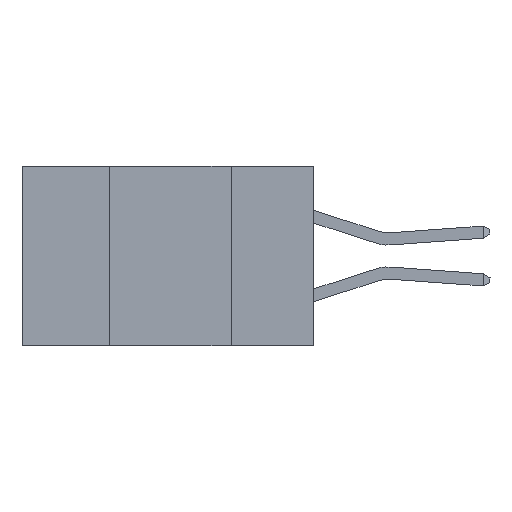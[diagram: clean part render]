
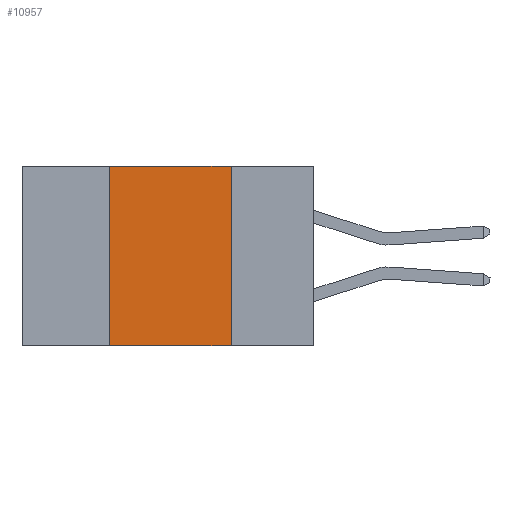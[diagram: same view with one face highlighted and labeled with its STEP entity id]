
A CAD part, left-side view. The second image highlights one B-rep face of the part: STEP entity #10957.
In plain terms, the highlighted planar face has unit normal (-1, 0, 0).
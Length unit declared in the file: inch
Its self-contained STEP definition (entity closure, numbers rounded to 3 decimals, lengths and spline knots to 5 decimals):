
#966 = DIRECTION ( 'NONE',  ( 0., 0., -1. ) ) ;
#1144 = ORIENTED_EDGE ( 'NONE', *, *, #2001, .F. ) ;
#1192 = AXIS2_PLACEMENT_3D ( 'NONE', #4629, #12158, #5756 ) ;
#1366 = CARTESIAN_POINT ( 'NONE',  ( 0., 0.6, 0. ) ) ;
#1712 = DIRECTION ( 'NONE',  ( 0., 0., 1. ) ) ;
#2001 = EDGE_CURVE ( 'NONE', #13180, #4942, #3575, .T. ) ;
#2554 = FACE_OUTER_BOUND ( 'NONE', #12454, .T. ) ;
#3108 = LINE ( 'NONE', #6059, #14188 ) ;
#3410 = VECTOR ( 'NONE', #3708, 39.37008 ) ;
#3421 = VERTEX_POINT ( 'NONE', #8029 ) ;
#3575 = LINE ( 'NONE', #8873, #12205 ) ;
#3578 = CARTESIAN_POINT ( 'NONE',  ( 0., 0.17, -0.37 ) ) ;
#3708 = DIRECTION ( 'NONE',  ( 0., -1., 0. ) ) ;
#3716 = ORIENTED_EDGE ( 'NONE', *, *, #11141, .T. ) ;
#4629 = CARTESIAN_POINT ( 'NONE',  ( 0., 0.6, 0. ) ) ;
#4942 = VERTEX_POINT ( 'NONE', #3578 ) ;
#5756 = DIRECTION ( 'NONE',  ( 0., 0., -1. ) ) ;
#6059 = CARTESIAN_POINT ( 'NONE',  ( 0., 0.6, -0.37 ) ) ;
#6244 = VECTOR ( 'NONE', #1712, 39.37008 ) ;
#6292 = CARTESIAN_POINT ( 'NONE',  ( 0., 0.42, 0. ) ) ;
#6396 = LINE ( 'NONE', #1366, #3410 ) ;
#7393 = CARTESIAN_POINT ( 'NONE',  ( 0., 0.17, 0. ) ) ;
#8029 = CARTESIAN_POINT ( 'NONE',  ( 0., 0.42, 0. ) ) ;
#8271 = DIRECTION ( 'NONE',  ( 0., -1., 0. ) ) ;
#8629 = CARTESIAN_POINT ( 'NONE',  ( 0., 0.42, -0.37 ) ) ;
#8873 = CARTESIAN_POINT ( 'NONE',  ( 0., 0.17, 0. ) ) ;
#9427 = EDGE_CURVE ( 'NONE', #3421, #13180, #6396, .T. ) ;
#9950 = ORIENTED_EDGE ( 'NONE', *, *, #11824, .F. ) ;
#10957 = ADVANCED_FACE ( 'NONE', ( #2554 ), #13155, .F. ) ;
#11141 = EDGE_CURVE ( 'NONE', #12559, #4942, #3108, .T. ) ;
#11578 = LINE ( 'NONE', #6292, #6244 ) ;
#11824 = EDGE_CURVE ( 'NONE', #12559, #3421, #11578, .T. ) ;
#12158 = DIRECTION ( 'NONE',  ( 1., 0., 0. ) ) ;
#12205 = VECTOR ( 'NONE', #966, 39.37008 ) ;
#12269 = ORIENTED_EDGE ( 'NONE', *, *, #9427, .F. ) ;
#12454 = EDGE_LOOP ( 'NONE', ( #1144, #12269, #9950, #3716 ) ) ;
#12559 = VERTEX_POINT ( 'NONE', #8629 ) ;
#13155 = PLANE ( 'NONE',  #1192 ) ;
#13180 = VERTEX_POINT ( 'NONE', #7393 ) ;
#14188 = VECTOR ( 'NONE', #8271, 39.37008 ) ;
